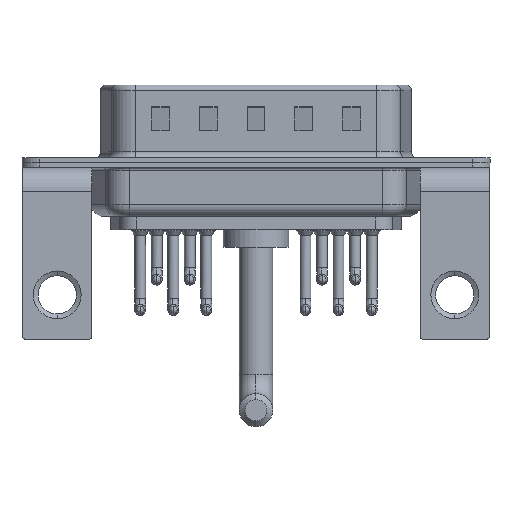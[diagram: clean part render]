
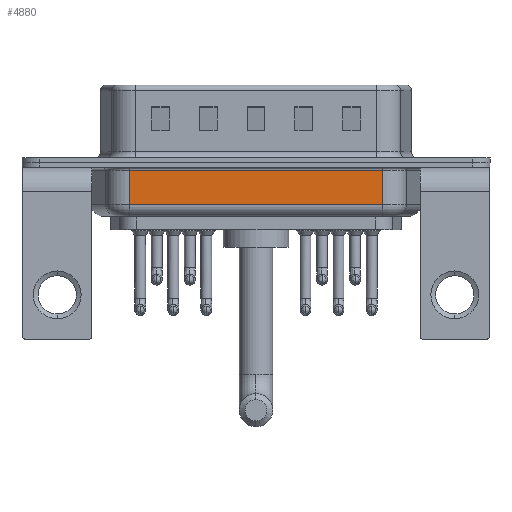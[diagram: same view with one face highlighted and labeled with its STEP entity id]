
A CAD part, front view. The second image highlights one B-rep face of the part: STEP entity #4880.
In plain terms, the highlighted planar face has unit normal (0, -1, 0).
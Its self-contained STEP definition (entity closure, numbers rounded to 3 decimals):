
#1587 = LINE ( 'NONE', #1801, #6952 ) ;
#1724 = DIRECTION ( 'NONE',  ( 0., 0., 1. ) ) ;
#1801 = CARTESIAN_POINT ( 'NONE',  ( 6.031, -5.35, -4.5 ) ) ;
#2865 = VERTEX_POINT ( 'NONE', #4349 ) ;
#3354 = DIRECTION ( 'NONE',  ( -1., 0., 0. ) ) ;
#3458 = DIRECTION ( 'NONE',  ( 0., 0., 1. ) ) ;
#4278 = CARTESIAN_POINT ( 'NONE',  ( 27.269, -5.35, -0.65 ) ) ;
#4349 = CARTESIAN_POINT ( 'NONE',  ( 27.269, -5.35, -3.5 ) ) ;
#4880 = ADVANCED_FACE ( 'NONE', ( #5261 ), #12365, .F. ) ;
#5020 = CARTESIAN_POINT ( 'NONE',  ( 6.031, -5.35, -3.5 ) ) ;
#5261 = FACE_OUTER_BOUND ( 'NONE', #22596, .T. ) ;
#5309 = EDGE_CURVE ( 'NONE', #10638, #18353, #7297, .T. ) ;
#5662 = CARTESIAN_POINT ( 'NONE',  ( 6.031, -5.35, -3.5 ) ) ;
#5737 = ORIENTED_EDGE ( 'NONE', *, *, #17779, .T. ) ;
#6499 = ORIENTED_EDGE ( 'NONE', *, *, #16074, .F. ) ;
#6952 = VECTOR ( 'NONE', #3458, 1000. ) ;
#7200 = VECTOR ( 'NONE', #23005, 1000. ) ;
#7297 = LINE ( 'NONE', #12226, #18831 ) ;
#7392 = CARTESIAN_POINT ( 'NONE',  ( 27.269, -5.35, -4.5 ) ) ;
#9341 = VERTEX_POINT ( 'NONE', #5662 ) ;
#10638 = VERTEX_POINT ( 'NONE', #4278 ) ;
#11006 = DIRECTION ( 'NONE',  ( 0., 0., 1. ) ) ;
#12080 = LINE ( 'NONE', #7392, #19331 ) ;
#12226 = CARTESIAN_POINT ( 'NONE',  ( 6.031, -5.35, -0.65 ) ) ;
#12365 = PLANE ( 'NONE',  #16601 ) ;
#13997 = LINE ( 'NONE', #5020, #7200 ) ;
#14236 = EDGE_CURVE ( 'NONE', #9341, #2865, #13997, .T. ) ;
#14355 = DIRECTION ( 'NONE',  ( 0., 1., 0. ) ) ;
#14518 = ORIENTED_EDGE ( 'NONE', *, *, #14236, .T. ) ;
#15980 = ORIENTED_EDGE ( 'NONE', *, *, #5309, .T. ) ;
#16074 = EDGE_CURVE ( 'NONE', #9341, #18353, #1587, .T. ) ;
#16601 = AXIS2_PLACEMENT_3D ( 'NONE', #21723, #14355, #1724 ) ;
#17666 = CARTESIAN_POINT ( 'NONE',  ( 6.031, -5.35, -0.65 ) ) ;
#17779 = EDGE_CURVE ( 'NONE', #2865, #10638, #12080, .T. ) ;
#18353 = VERTEX_POINT ( 'NONE', #17666 ) ;
#18831 = VECTOR ( 'NONE', #3354, 1000. ) ;
#19331 = VECTOR ( 'NONE', #11006, 1000. ) ;
#21723 = CARTESIAN_POINT ( 'NONE',  ( 6.031, -5.35, -4.5 ) ) ;
#22596 = EDGE_LOOP ( 'NONE', ( #6499, #14518, #5737, #15980 ) ) ;
#23005 = DIRECTION ( 'NONE',  ( 1., 0., 0. ) ) ;
